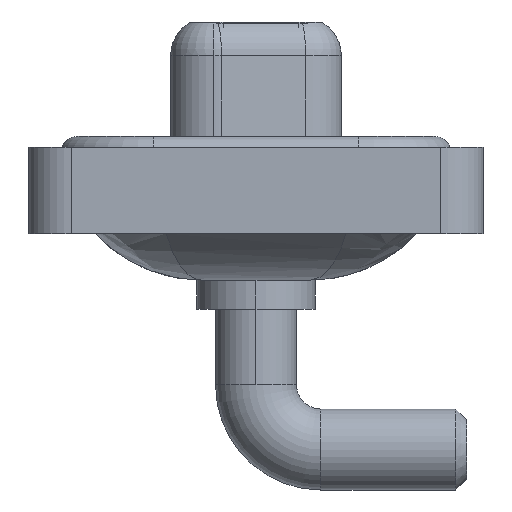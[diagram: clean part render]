
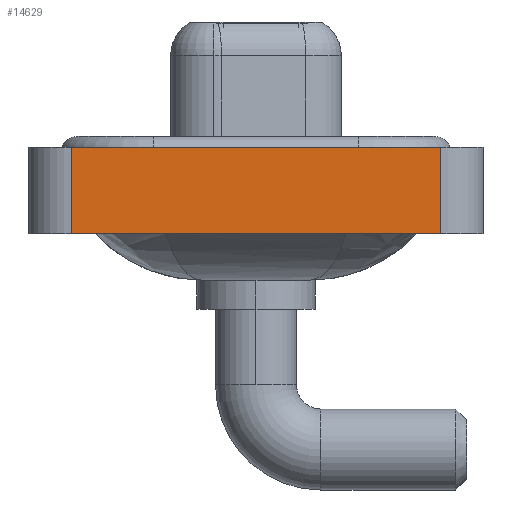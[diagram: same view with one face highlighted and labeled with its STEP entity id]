
A CAD part, left-side view. The second image highlights one B-rep face of the part: STEP entity #14629.
In plain terms, the highlighted planar face has unit normal (-1, 0, 0).
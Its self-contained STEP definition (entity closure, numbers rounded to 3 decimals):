
#293 = DIRECTION ( 'NONE',  ( 0., -1., 0. ) ) ;
#2145 = CARTESIAN_POINT ( 'NONE',  ( -7.35, -8.55, 0.4 ) ) ;
#2250 = LINE ( 'NONE', #11040, #6280 ) ;
#2655 = ORIENTED_EDGE ( 'NONE', *, *, #15001, .T. ) ;
#2995 = CARTESIAN_POINT ( 'NONE',  ( -7.35, 8.55, 0.4 ) ) ;
#3776 = CARTESIAN_POINT ( 'NONE',  ( -7.35, -8.55, 0.4 ) ) ;
#5306 = VERTEX_POINT ( 'NONE', #11058 ) ;
#5608 = VERTEX_POINT ( 'NONE', #8966 ) ;
#5614 = PLANE ( 'NONE',  #13657 ) ;
#6205 = DIRECTION ( 'NONE',  ( 0., 0., 1. ) ) ;
#6280 = VECTOR ( 'NONE', #7338, 1000. ) ;
#6342 = ORIENTED_EDGE ( 'NONE', *, *, #11198, .T. ) ;
#7338 = DIRECTION ( 'NONE',  ( 0., 0., 1. ) ) ;
#7625 = LINE ( 'NONE', #3776, #10487 ) ;
#8734 = EDGE_CURVE ( 'NONE', #5608, #8969, #2250, .T. ) ;
#8792 = CARTESIAN_POINT ( 'NONE',  ( -7.35, -8.55, -3.6 ) ) ;
#8966 = CARTESIAN_POINT ( 'NONE',  ( -7.35, 8.55, -3.6 ) ) ;
#8968 = LINE ( 'NONE', #8792, #12413 ) ;
#8969 = VERTEX_POINT ( 'NONE', #2995 ) ;
#9452 = ORIENTED_EDGE ( 'NONE', *, *, #8734, .F. ) ;
#10017 = CARTESIAN_POINT ( 'NONE',  ( -7.35, -8.55, -3.6 ) ) ;
#10487 = VECTOR ( 'NONE', #293, 1000. ) ;
#11040 = CARTESIAN_POINT ( 'NONE',  ( -7.35, 8.55, -3.6 ) ) ;
#11058 = CARTESIAN_POINT ( 'NONE',  ( -7.35, -8.55, -3.6 ) ) ;
#11198 = EDGE_CURVE ( 'NONE', #5608, #5306, #8968, .T. ) ;
#11743 = DIRECTION ( 'NONE',  ( -1., 0., 0. ) ) ;
#12413 = VECTOR ( 'NONE', #14010, 1000. ) ;
#12506 = LINE ( 'NONE', #10017, #14392 ) ;
#13244 = DIRECTION ( 'NONE',  ( 0., 0., 1. ) ) ;
#13657 = AXIS2_PLACEMENT_3D ( 'NONE', #15636, #11743, #13244 ) ;
#14010 = DIRECTION ( 'NONE',  ( 0., -1., 0. ) ) ;
#14181 = EDGE_LOOP ( 'NONE', ( #2655, #14877, #9452, #6342 ) ) ;
#14392 = VECTOR ( 'NONE', #6205, 1000. ) ;
#14629 = ADVANCED_FACE ( 'NONE', ( #14640 ), #5614, .T. ) ;
#14640 = FACE_OUTER_BOUND ( 'NONE', #14181, .T. ) ;
#14877 = ORIENTED_EDGE ( 'NONE', *, *, #14945, .F. ) ;
#14945 = EDGE_CURVE ( 'NONE', #8969, #16303, #7625, .T. ) ;
#15001 = EDGE_CURVE ( 'NONE', #5306, #16303, #12506, .T. ) ;
#15636 = CARTESIAN_POINT ( 'NONE',  ( -7.35, -8.55, -3.6 ) ) ;
#16303 = VERTEX_POINT ( 'NONE', #2145 ) ;
